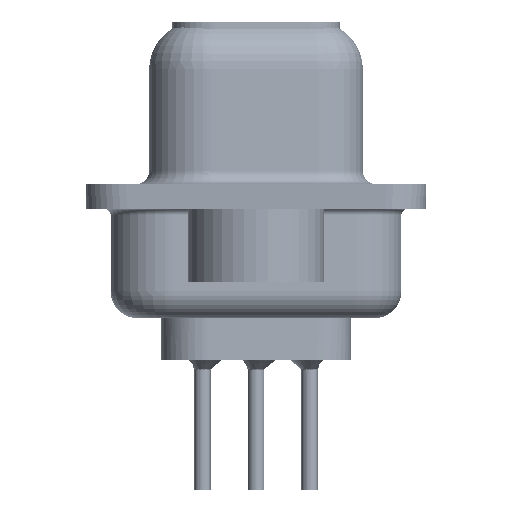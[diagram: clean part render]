
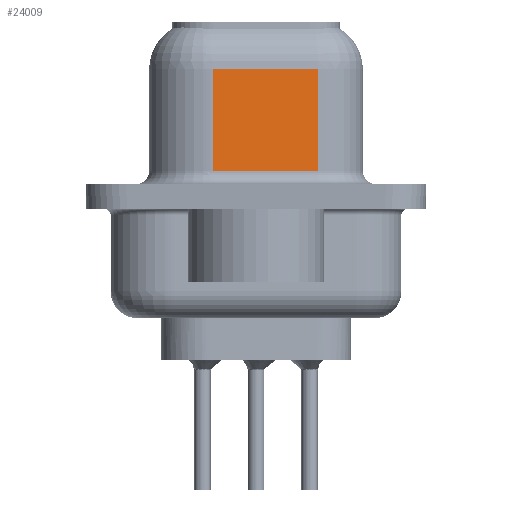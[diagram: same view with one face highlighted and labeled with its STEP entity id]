
A CAD part, left-side view. The second image highlights one B-rep face of the part: STEP entity #24009.
In plain terms, the highlighted planar face has unit normal (-0.985, -0.174, 0).
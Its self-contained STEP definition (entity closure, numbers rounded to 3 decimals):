
#190 = CARTESIAN_POINT ( 'NONE',  ( 5.053, -2.297, 4.7 ) ) ;
#873 = EDGE_LOOP ( 'NONE', ( #22770, #30328, #30002, #15449 ) ) ;
#1481 = CARTESIAN_POINT ( 'NONE',  ( 5.053, -2.297, 0.95 ) ) ;
#2665 = EDGE_CURVE ( 'NONE', #16838, #32414, #4529, .T. ) ;
#2688 = CARTESIAN_POINT ( 'NONE',  ( 4.365, 1.603, 6.45 ) ) ;
#4529 = LINE ( 'NONE', #190, #19061 ) ;
#4699 = LINE ( 'NONE', #2688, #20984 ) ;
#6933 = LINE ( 'NONE', #32390, #31385 ) ;
#7095 = DIRECTION ( 'NONE',  ( 0., 0., -1. ) ) ;
#7354 = DIRECTION ( 'NONE',  ( 0., 0., -1. ) ) ;
#8565 = DIRECTION ( 'NONE',  ( -0.174, 0.985, 0. ) ) ;
#12171 = DIRECTION ( 'NONE',  ( -0.174, 0.985, 0. ) ) ;
#13228 = VECTOR ( 'NONE', #28889, 1000. ) ;
#13540 = CARTESIAN_POINT ( 'NONE',  ( 5.053, -2.297, 6.45 ) ) ;
#14464 = CARTESIAN_POINT ( 'NONE',  ( 4.365, 1.603, 4.7 ) ) ;
#14517 = EDGE_CURVE ( 'NONE', #15119, #18637, #31230, .T. ) ;
#15119 = VERTEX_POINT ( 'NONE', #18635 ) ;
#15449 = ORIENTED_EDGE ( 'NONE', *, *, #14517, .T. ) ;
#16139 = AXIS2_PLACEMENT_3D ( 'NONE', #13540, #31354, #8565 ) ;
#16838 = VERTEX_POINT ( 'NONE', #25624 ) ;
#17969 = EDGE_CURVE ( 'NONE', #16838, #18637, #6933, .T. ) ;
#18635 = CARTESIAN_POINT ( 'NONE',  ( 4.365, 1.603, 0.95 ) ) ;
#18637 = VERTEX_POINT ( 'NONE', #23769 ) ;
#19061 = VECTOR ( 'NONE', #12171, 1000. ) ;
#20984 = VECTOR ( 'NONE', #7354, 1000. ) ;
#22770 = ORIENTED_EDGE ( 'NONE', *, *, #17969, .F. ) ;
#23188 = PLANE ( 'NONE',  #16139 ) ;
#23769 = CARTESIAN_POINT ( 'NONE',  ( 5.053, -2.297, 0.95 ) ) ;
#24009 = ADVANCED_FACE ( 'NONE', ( #28515 ), #23188, .F. ) ;
#25624 = CARTESIAN_POINT ( 'NONE',  ( 5.053, -2.297, 4.7 ) ) ;
#25723 = EDGE_CURVE ( 'NONE', #32414, #15119, #4699, .T. ) ;
#28515 = FACE_OUTER_BOUND ( 'NONE', #873, .T. ) ;
#28889 = DIRECTION ( 'NONE',  ( 0.174, -0.985, 0. ) ) ;
#30002 = ORIENTED_EDGE ( 'NONE', *, *, #25723, .T. ) ;
#30328 = ORIENTED_EDGE ( 'NONE', *, *, #2665, .T. ) ;
#31230 = LINE ( 'NONE', #1481, #13228 ) ;
#31354 = DIRECTION ( 'NONE',  ( 0.985, 0.174, 0. ) ) ;
#31385 = VECTOR ( 'NONE', #7095, 1000. ) ;
#32390 = CARTESIAN_POINT ( 'NONE',  ( 5.053, -2.297, 6.45 ) ) ;
#32414 = VERTEX_POINT ( 'NONE', #14464 ) ;
